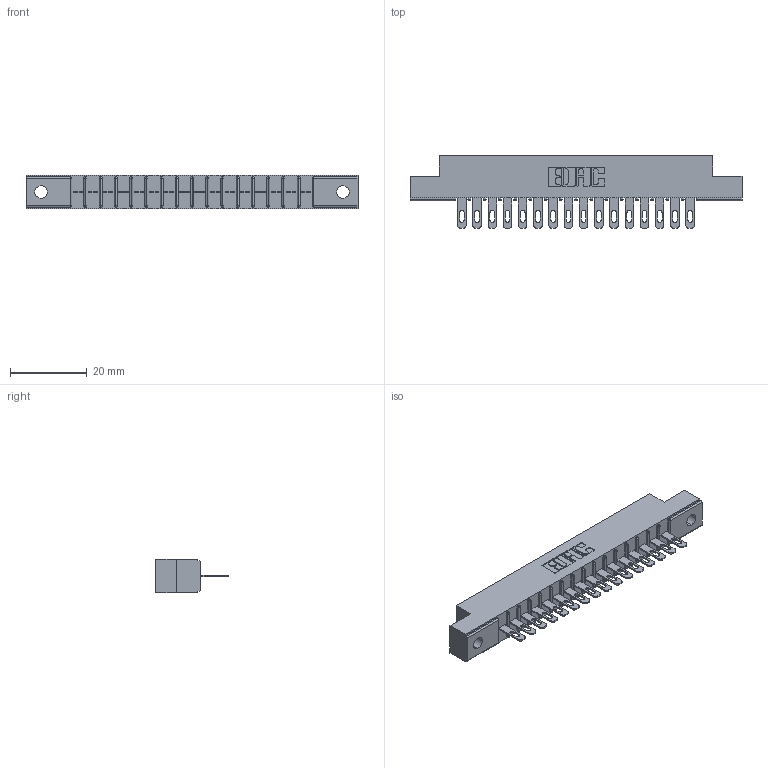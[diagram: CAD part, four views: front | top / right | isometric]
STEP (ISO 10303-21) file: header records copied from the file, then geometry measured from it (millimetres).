
FILE_DESCRIPTION (( 'STEP AP203' ), '1' );
FILE_NAME ('306-016-500-102.STEP', '2019-09-11T20:02:11', ( '' ), ( '' ), 'SwSTEP 2.0', 'SolidWorks 2016', '' );
FILE_SCHEMA (( 'CONFIG_CONTROL_DESIGN' ));
Length unit declared in the file: inch
Products named in the file (3): 306-290-001_100; 306 Part_.128 Dia; 306-016-500-102
Assembly tree (17 placements, depth 2):
  306-016-500-102
    306 Part_.128 Dia
    306-290-001_100  x16
Bounding box: 86.41 x 18.87 x 8.71 mm (x, y, z)
Volume: 5894.1 mm3; surface area: 8528 mm2
Topology: 17 solids, 17 shells, 1332 faces, 3756 edges, 2416 vertices
Faces by surface type: plane 868, cylinder 400, sphere 64
Entity records: 18455 total; most frequent: CARTESIAN_POINT 3095, ORIENTED_EDGE 3064, DIRECTION 3056, EDGE_CURVE 1532, VECTOR 1182, LINE 1182, VERTEX_POINT 976, AXIS2_PLACEMENT_3D 937
